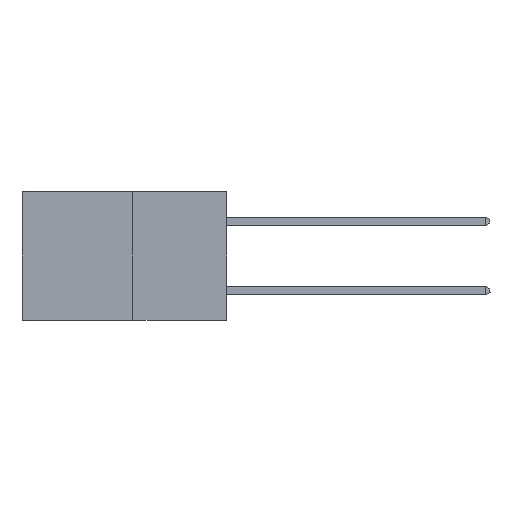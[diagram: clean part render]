
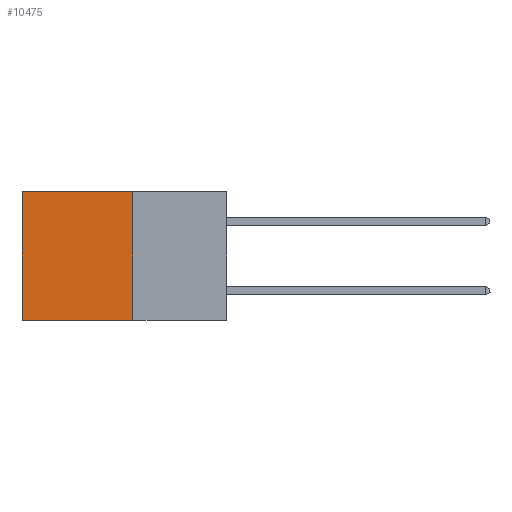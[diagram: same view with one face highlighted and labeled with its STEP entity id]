
A CAD part, left-side view. The second image highlights one B-rep face of the part: STEP entity #10475.
In plain terms, the highlighted planar face has unit normal (-1, 0, 0).
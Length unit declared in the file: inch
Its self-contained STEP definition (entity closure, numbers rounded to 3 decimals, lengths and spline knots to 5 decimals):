
#161 = VECTOR ( 'NONE', #2528, 39.37008 ) ;
#449 = DIRECTION ( 'NONE',  ( 0., 1., 0. ) ) ;
#799 = AXIS2_PLACEMENT_3D ( 'NONE', #9914, #2358, #11198 ) ;
#994 = EDGE_CURVE ( 'NONE', #5653, #10730, #14690, .T. ) ;
#1099 = PLANE ( 'NONE',  #799 ) ;
#1206 = CARTESIAN_POINT ( 'NONE',  ( 0.277, 0.27, -0.37 ) ) ;
#1288 = VECTOR ( 'NONE', #449, 39.37008 ) ;
#1399 = VERTEX_POINT ( 'NONE', #2467 ) ;
#1428 = EDGE_CURVE ( 'NONE', #1399, #10730, #7226, .T. ) ;
#2358 = DIRECTION ( 'NONE',  ( 1., 0., 0. ) ) ;
#2396 = LINE ( 'NONE', #10678, #5344 ) ;
#2467 = CARTESIAN_POINT ( 'NONE',  ( 0.277, 0.59, 0. ) ) ;
#2528 = DIRECTION ( 'NONE',  ( 0., 0., -1. ) ) ;
#3230 = DIRECTION ( 'NONE',  ( 0., 0., -1. ) ) ;
#3567 = CARTESIAN_POINT ( 'NONE',  ( 0.277, 0.27, 0. ) ) ;
#3724 = ORIENTED_EDGE ( 'NONE', *, *, #994, .F. ) ;
#5299 = EDGE_LOOP ( 'NONE', ( #15059, #3724, #15710, #7004 ) ) ;
#5344 = VECTOR ( 'NONE', #10635, 39.37008 ) ;
#5653 = VERTEX_POINT ( 'NONE', #1206 ) ;
#6663 = LINE ( 'NONE', #14568, #13397 ) ;
#7004 = ORIENTED_EDGE ( 'NONE', *, *, #7322, .T. ) ;
#7226 = LINE ( 'NONE', #13874, #161 ) ;
#7322 = EDGE_CURVE ( 'NONE', #9187, #1399, #2396, .T. ) ;
#9187 = VERTEX_POINT ( 'NONE', #3567 ) ;
#9914 = CARTESIAN_POINT ( 'NONE',  ( 0.277, 0.27, -0.37 ) ) ;
#10475 = ADVANCED_FACE ( 'NONE', ( #12426 ), #1099, .F. ) ;
#10526 = CARTESIAN_POINT ( 'NONE',  ( 0.277, 0.27, -0.37 ) ) ;
#10635 = DIRECTION ( 'NONE',  ( 0., 1., 0. ) ) ;
#10678 = CARTESIAN_POINT ( 'NONE',  ( 0.277, 0.27, 0. ) ) ;
#10730 = VERTEX_POINT ( 'NONE', #14087 ) ;
#11198 = DIRECTION ( 'NONE',  ( 0., 0., -1. ) ) ;
#12426 = FACE_OUTER_BOUND ( 'NONE', #5299, .T. ) ;
#13397 = VECTOR ( 'NONE', #3230, 39.37008 ) ;
#13874 = CARTESIAN_POINT ( 'NONE',  ( 0.277, 0.59, -0.37 ) ) ;
#14087 = CARTESIAN_POINT ( 'NONE',  ( 0.277, 0.59, -0.37 ) ) ;
#14568 = CARTESIAN_POINT ( 'NONE',  ( 0.277, 0.27, -0.37 ) ) ;
#14690 = LINE ( 'NONE', #10526, #1288 ) ;
#15059 = ORIENTED_EDGE ( 'NONE', *, *, #1428, .T. ) ;
#15686 = EDGE_CURVE ( 'NONE', #9187, #5653, #6663, .T. ) ;
#15710 = ORIENTED_EDGE ( 'NONE', *, *, #15686, .F. ) ;
